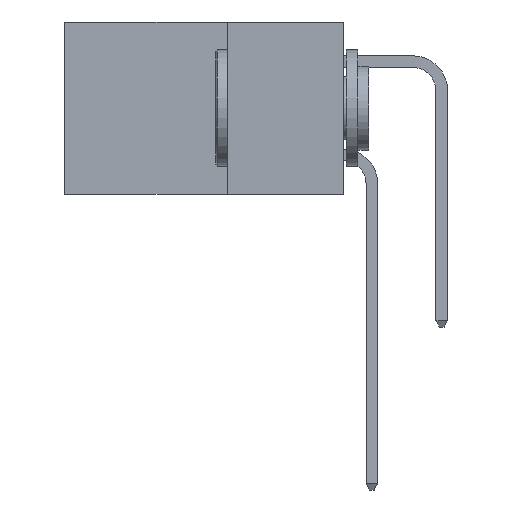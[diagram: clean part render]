
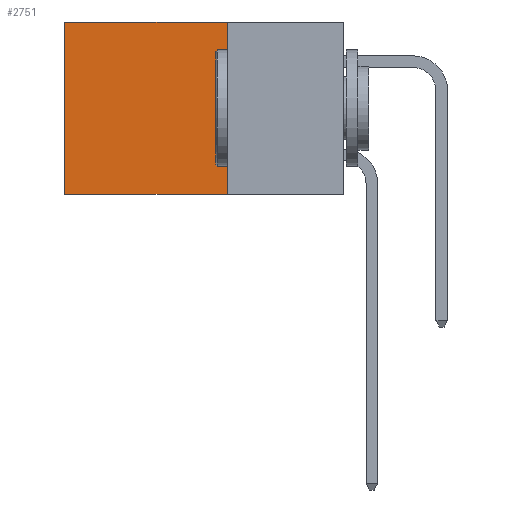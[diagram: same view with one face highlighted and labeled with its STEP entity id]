
A CAD part, left-side view. The second image highlights one B-rep face of the part: STEP entity #2751.
In plain terms, the highlighted planar face has unit normal (-1, 0, 0).
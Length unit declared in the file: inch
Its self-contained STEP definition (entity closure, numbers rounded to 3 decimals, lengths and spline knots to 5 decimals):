
#309 = CARTESIAN_POINT ( 'NONE',  ( 0.2615, 0.25, -0.37 ) ) ;
#776 = EDGE_CURVE ( 'NONE', #8152, #11493, #9260, .T. ) ;
#1201 = DIRECTION ( 'NONE',  ( 0., 0., -1. ) ) ;
#1222 = DIRECTION ( 'NONE',  ( 0., 0., -1. ) ) ;
#1247 = CARTESIAN_POINT ( 'NONE',  ( 0.2615, 0.6, -0.37 ) ) ;
#1557 = CARTESIAN_POINT ( 'NONE',  ( 0.2615, 0.25, -0.37 ) ) ;
#2370 = CARTESIAN_POINT ( 'NONE',  ( 0.2615, 0.25, -0.37 ) ) ;
#2630 = AXIS2_PLACEMENT_3D ( 'NONE', #14340, #17423, #14724 ) ;
#2751 = ADVANCED_FACE ( 'NONE', ( #11123 ), #14333, .F. ) ;
#3981 = LINE ( 'NONE', #309, #7736 ) ;
#4145 = EDGE_LOOP ( 'NONE', ( #6564, #16330, #17204, #11671 ) ) ;
#4317 = VECTOR ( 'NONE', #15344, 39.37008 ) ;
#4771 = LINE ( 'NONE', #8333, #4317 ) ;
#5080 = VERTEX_POINT ( 'NONE', #10275 ) ;
#5236 = CARTESIAN_POINT ( 'NONE',  ( 0.2615, 0.25, 0. ) ) ;
#6218 = EDGE_CURVE ( 'NONE', #11493, #14829, #3981, .T. ) ;
#6564 = ORIENTED_EDGE ( 'NONE', *, *, #8514, .T. ) ;
#7736 = VECTOR ( 'NONE', #18163, 39.37008 ) ;
#8152 = VERTEX_POINT ( 'NONE', #5236 ) ;
#8333 = CARTESIAN_POINT ( 'NONE',  ( 0.2615, 0.25, 0. ) ) ;
#8514 = EDGE_CURVE ( 'NONE', #5080, #14829, #17199, .T. ) ;
#8807 = VECTOR ( 'NONE', #1222, 39.37008 ) ;
#9260 = LINE ( 'NONE', #1557, #8807 ) ;
#10275 = CARTESIAN_POINT ( 'NONE',  ( 0.2615, 0.6, 0. ) ) ;
#10928 = CARTESIAN_POINT ( 'NONE',  ( 0.2615, 0.6, -0.37 ) ) ;
#11123 = FACE_OUTER_BOUND ( 'NONE', #4145, .T. ) ;
#11493 = VERTEX_POINT ( 'NONE', #2370 ) ;
#11671 = ORIENTED_EDGE ( 'NONE', *, *, #14932, .T. ) ;
#14333 = PLANE ( 'NONE',  #2630 ) ;
#14340 = CARTESIAN_POINT ( 'NONE',  ( 0.2615, 0.25, -0.37 ) ) ;
#14724 = DIRECTION ( 'NONE',  ( 0., 0., -1. ) ) ;
#14829 = VERTEX_POINT ( 'NONE', #10928 ) ;
#14932 = EDGE_CURVE ( 'NONE', #8152, #5080, #4771, .T. ) ;
#15344 = DIRECTION ( 'NONE',  ( 0., 1., 0. ) ) ;
#16330 = ORIENTED_EDGE ( 'NONE', *, *, #6218, .F. ) ;
#16785 = VECTOR ( 'NONE', #1201, 39.37008 ) ;
#17199 = LINE ( 'NONE', #1247, #16785 ) ;
#17204 = ORIENTED_EDGE ( 'NONE', *, *, #776, .F. ) ;
#17423 = DIRECTION ( 'NONE',  ( 1., 0., 0. ) ) ;
#18163 = DIRECTION ( 'NONE',  ( 0., 1., 0. ) ) ;
